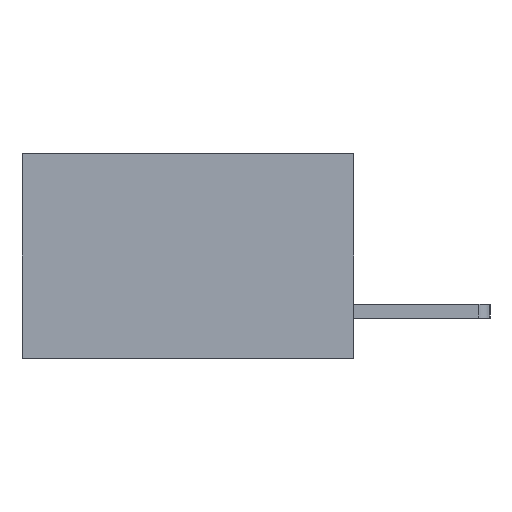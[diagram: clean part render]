
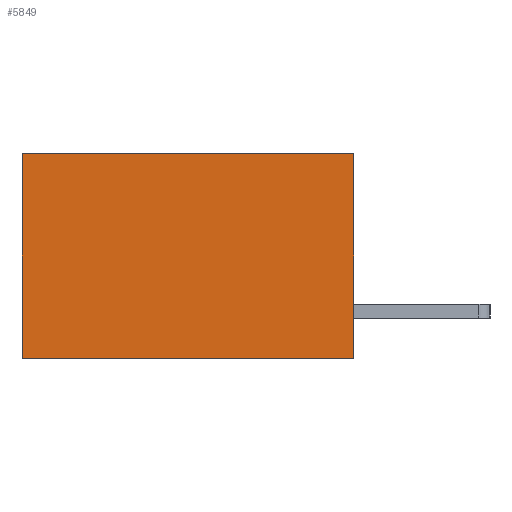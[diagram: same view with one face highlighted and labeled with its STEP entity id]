
A CAD part, left-side view. The second image highlights one B-rep face of the part: STEP entity #5849.
In plain terms, the highlighted planar face has unit normal (-1, 0, 0).
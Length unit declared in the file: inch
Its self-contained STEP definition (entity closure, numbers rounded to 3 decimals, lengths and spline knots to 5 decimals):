
#379 = AXIS2_PLACEMENT_3D ( 'NONE', #6885, #2288, #12547 ) ;
#608 = ORIENTED_EDGE ( 'NONE', *, *, #7696, .F. ) ;
#1851 = LINE ( 'NONE', #12193, #3192 ) ;
#2222 = FACE_OUTER_BOUND ( 'NONE', #8462, .T. ) ;
#2288 = DIRECTION ( 'NONE',  ( 1., 0., 0. ) ) ;
#2625 = VECTOR ( 'NONE', #2975, 39.37008 ) ;
#2975 = DIRECTION ( 'NONE',  ( 0., 1., 0. ) ) ;
#3192 = VECTOR ( 'NONE', #11706, 39.37008 ) ;
#3639 = VERTEX_POINT ( 'NONE', #11350 ) ;
#3839 = CARTESIAN_POINT ( 'NONE',  ( 0.2875, 0.6, 0. ) ) ;
#5636 = EDGE_CURVE ( 'NONE', #3639, #7065, #1851, .T. ) ;
#5849 = ADVANCED_FACE ( 'NONE', ( #2222 ), #7847, .F. ) ;
#5872 = DIRECTION ( 'NONE',  ( 0., 0., -1. ) ) ;
#6885 = CARTESIAN_POINT ( 'NONE',  ( 0.2875, 0., 0. ) ) ;
#7065 = VERTEX_POINT ( 'NONE', #10130 ) ;
#7222 = EDGE_CURVE ( 'NONE', #7537, #7065, #12423, .T. ) ;
#7532 = CARTESIAN_POINT ( 'NONE',  ( 0.2875, 0., 0. ) ) ;
#7537 = VERTEX_POINT ( 'NONE', #3839 ) ;
#7556 = CARTESIAN_POINT ( 'NONE',  ( 0.2875, 0., 0. ) ) ;
#7589 = LINE ( 'NONE', #10830, #8557 ) ;
#7696 = EDGE_CURVE ( 'NONE', #10344, #3639, #7589, .T. ) ;
#7847 = PLANE ( 'NONE',  #379 ) ;
#8076 = CARTESIAN_POINT ( 'NONE',  ( 0.2875, 0.6, 0. ) ) ;
#8419 = ORIENTED_EDGE ( 'NONE', *, *, #5636, .F. ) ;
#8462 = EDGE_LOOP ( 'NONE', ( #13063, #8419, #608, #10107 ) ) ;
#8557 = VECTOR ( 'NONE', #13046, 39.37008 ) ;
#9166 = VECTOR ( 'NONE', #5872, 39.37008 ) ;
#10107 = ORIENTED_EDGE ( 'NONE', *, *, #11642, .T. ) ;
#10130 = CARTESIAN_POINT ( 'NONE',  ( 0.2875, 0.6, -0.37 ) ) ;
#10344 = VERTEX_POINT ( 'NONE', #7532 ) ;
#10830 = CARTESIAN_POINT ( 'NONE',  ( 0.2875, 0., 0. ) ) ;
#11350 = CARTESIAN_POINT ( 'NONE',  ( 0.2875, 0., -0.37 ) ) ;
#11642 = EDGE_CURVE ( 'NONE', #10344, #7537, #13238, .T. ) ;
#11706 = DIRECTION ( 'NONE',  ( 0., 1., 0. ) ) ;
#12193 = CARTESIAN_POINT ( 'NONE',  ( 0.2875, 0., -0.37 ) ) ;
#12423 = LINE ( 'NONE', #8076, #9166 ) ;
#12547 = DIRECTION ( 'NONE',  ( 0., 0., -1. ) ) ;
#13046 = DIRECTION ( 'NONE',  ( 0., 0., -1. ) ) ;
#13063 = ORIENTED_EDGE ( 'NONE', *, *, #7222, .T. ) ;
#13238 = LINE ( 'NONE', #7556, #2625 ) ;
